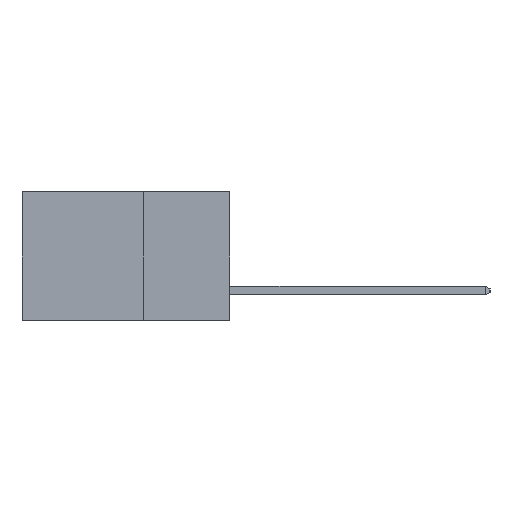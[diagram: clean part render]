
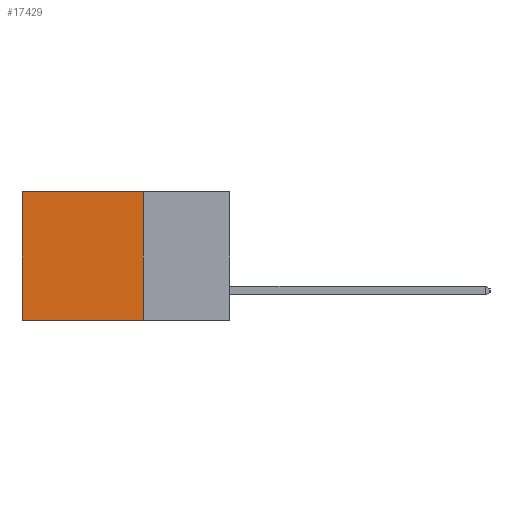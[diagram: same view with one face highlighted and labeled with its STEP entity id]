
A CAD part, left-side view. The second image highlights one B-rep face of the part: STEP entity #17429.
In plain terms, the highlighted planar face has unit normal (-1, 0, 0).
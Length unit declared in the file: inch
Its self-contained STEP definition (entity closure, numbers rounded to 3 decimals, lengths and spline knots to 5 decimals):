
#1133 = DIRECTION ( 'NONE',  ( 0., 0., -1. ) ) ;
#1859 = EDGE_CURVE ( 'NONE', #8675, #17110, #15941, .T. ) ;
#2174 = VERTEX_POINT ( 'NONE', #15193 ) ;
#3780 = CARTESIAN_POINT ( 'NONE',  ( 0.2615, 0.25, -0.37 ) ) ;
#4053 = VECTOR ( 'NONE', #18712, 39.37008 ) ;
#4544 = FACE_OUTER_BOUND ( 'NONE', #18564, .T. ) ;
#4907 = VECTOR ( 'NONE', #6147, 39.37008 ) ;
#6050 = ORIENTED_EDGE ( 'NONE', *, *, #12397, .T. ) ;
#6147 = DIRECTION ( 'NONE',  ( 0., 0., -1. ) ) ;
#6365 = CARTESIAN_POINT ( 'NONE',  ( 0.2615, 0.25, 0. ) ) ;
#6471 = LINE ( 'NONE', #6365, #13889 ) ;
#7395 = CARTESIAN_POINT ( 'NONE',  ( 0.2615, 0.6, 0. ) ) ;
#8675 = VERTEX_POINT ( 'NONE', #3780 ) ;
#9496 = LINE ( 'NONE', #15001, #4907 ) ;
#10370 = EDGE_CURVE ( 'NONE', #14888, #17110, #15352, .T. ) ;
#10372 = ORIENTED_EDGE ( 'NONE', *, *, #14154, .F. ) ;
#10470 = DIRECTION ( 'NONE',  ( 1., 0., 0. ) ) ;
#10578 = DIRECTION ( 'NONE',  ( 0., 0., -1. ) ) ;
#11186 = ORIENTED_EDGE ( 'NONE', *, *, #10370, .T. ) ;
#11264 = CARTESIAN_POINT ( 'NONE',  ( 0.2615, 0.6, -0.37 ) ) ;
#11518 = VECTOR ( 'NONE', #10578, 39.37008 ) ;
#12397 = EDGE_CURVE ( 'NONE', #2174, #14888, #6471, .T. ) ;
#13889 = VECTOR ( 'NONE', #18053, 39.37008 ) ;
#14154 = EDGE_CURVE ( 'NONE', #2174, #8675, #9496, .T. ) ;
#14775 = CARTESIAN_POINT ( 'NONE',  ( 0.2615, 0.25, -0.37 ) ) ;
#14867 = CARTESIAN_POINT ( 'NONE',  ( 0.2615, 0.6, -0.37 ) ) ;
#14888 = VERTEX_POINT ( 'NONE', #7395 ) ;
#15001 = CARTESIAN_POINT ( 'NONE',  ( 0.2615, 0.25, -0.37 ) ) ;
#15071 = ORIENTED_EDGE ( 'NONE', *, *, #1859, .F. ) ;
#15193 = CARTESIAN_POINT ( 'NONE',  ( 0.2615, 0.25, 0. ) ) ;
#15352 = LINE ( 'NONE', #14867, #11518 ) ;
#15941 = LINE ( 'NONE', #18729, #4053 ) ;
#17110 = VERTEX_POINT ( 'NONE', #11264 ) ;
#17128 = AXIS2_PLACEMENT_3D ( 'NONE', #14775, #10470, #1133 ) ;
#17429 = ADVANCED_FACE ( 'NONE', ( #4544 ), #19069, .F. ) ;
#18053 = DIRECTION ( 'NONE',  ( 0., 1., 0. ) ) ;
#18564 = EDGE_LOOP ( 'NONE', ( #11186, #15071, #10372, #6050 ) ) ;
#18712 = DIRECTION ( 'NONE',  ( 0., 1., 0. ) ) ;
#18729 = CARTESIAN_POINT ( 'NONE',  ( 0.2615, 0.25, -0.37 ) ) ;
#19069 = PLANE ( 'NONE',  #17128 ) ;
